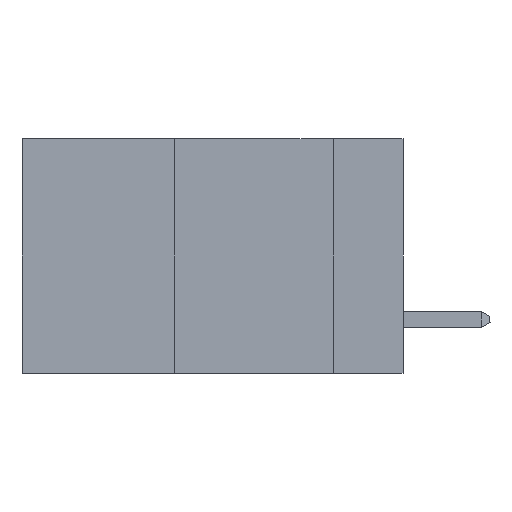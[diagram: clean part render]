
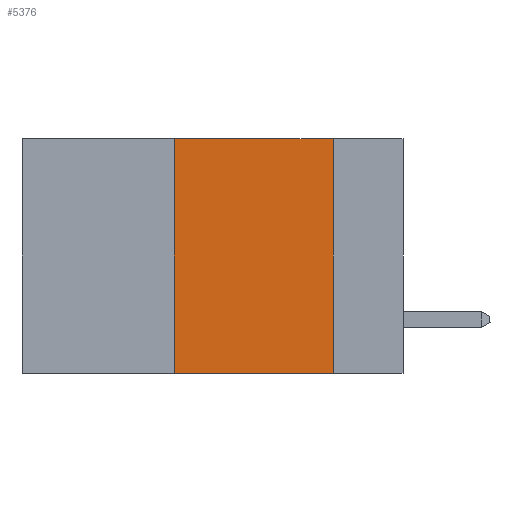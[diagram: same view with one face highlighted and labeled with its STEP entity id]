
A CAD part, left-side view. The second image highlights one B-rep face of the part: STEP entity #5376.
In plain terms, the highlighted planar face has unit normal (-1, 0, 0).
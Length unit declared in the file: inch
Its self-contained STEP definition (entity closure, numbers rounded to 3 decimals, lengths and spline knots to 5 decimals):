
#1169 = AXIS2_PLACEMENT_3D ( 'NONE', #4133, #14117, #9190 ) ;
#1533 = CARTESIAN_POINT ( 'NONE',  ( 0., 0.6, 0. ) ) ;
#1598 = VECTOR ( 'NONE', #25579, 39.37008 ) ;
#3193 = ORIENTED_EDGE ( 'NONE', *, *, #7996, .F. ) ;
#4133 = CARTESIAN_POINT ( 'NONE',  ( 0., 0.6, 0. ) ) ;
#5376 = ADVANCED_FACE ( 'NONE', ( #31578 ), #29357, .F. ) ;
#5491 = LINE ( 'NONE', #19817, #31745 ) ;
#7757 = CARTESIAN_POINT ( 'NONE',  ( 0., 0.36, 0. ) ) ;
#7996 = EDGE_CURVE ( 'NONE', #14707, #30590, #23059, .T. ) ;
#8188 = ORIENTED_EDGE ( 'NONE', *, *, #14630, .F. ) ;
#8896 = EDGE_CURVE ( 'NONE', #24119, #30255, #5491, .T. ) ;
#9190 = DIRECTION ( 'NONE',  ( 0., 0., -1. ) ) ;
#11296 = VECTOR ( 'NONE', #16432, 39.37008 ) ;
#12217 = ORIENTED_EDGE ( 'NONE', *, *, #16484, .T. ) ;
#12591 = DIRECTION ( 'NONE',  ( 0., -1., 0. ) ) ;
#13090 = CARTESIAN_POINT ( 'NONE',  ( 0., 0.36, 0. ) ) ;
#14106 = CARTESIAN_POINT ( 'NONE',  ( 0., 0.11, -0.37 ) ) ;
#14117 = DIRECTION ( 'NONE',  ( 1., 0., 0. ) ) ;
#14630 = EDGE_CURVE ( 'NONE', #30590, #24119, #18474, .T. ) ;
#14707 = VERTEX_POINT ( 'NONE', #19080 ) ;
#16432 = DIRECTION ( 'NONE',  ( 0., -1., 0. ) ) ;
#16484 = EDGE_CURVE ( 'NONE', #14707, #30255, #20738, .T. ) ;
#17288 = CARTESIAN_POINT ( 'NONE',  ( 0., 0.6, -0.37 ) ) ;
#18243 = ORIENTED_EDGE ( 'NONE', *, *, #8896, .F. ) ;
#18474 = LINE ( 'NONE', #1533, #11296 ) ;
#19080 = CARTESIAN_POINT ( 'NONE',  ( 0., 0.36, -0.37 ) ) ;
#19557 = EDGE_LOOP ( 'NONE', ( #18243, #8188, #3193, #12217 ) ) ;
#19817 = CARTESIAN_POINT ( 'NONE',  ( 0., 0.11, 0. ) ) ;
#20738 = LINE ( 'NONE', #17288, #24754 ) ;
#23059 = LINE ( 'NONE', #7757, #1598 ) ;
#23729 = CARTESIAN_POINT ( 'NONE',  ( 0., 0.11, 0. ) ) ;
#24119 = VERTEX_POINT ( 'NONE', #23729 ) ;
#24754 = VECTOR ( 'NONE', #12591, 39.37008 ) ;
#25579 = DIRECTION ( 'NONE',  ( 0., 0., 1. ) ) ;
#29191 = DIRECTION ( 'NONE',  ( 0., 0., -1. ) ) ;
#29357 = PLANE ( 'NONE',  #1169 ) ;
#30255 = VERTEX_POINT ( 'NONE', #14106 ) ;
#30590 = VERTEX_POINT ( 'NONE', #13090 ) ;
#31578 = FACE_OUTER_BOUND ( 'NONE', #19557, .T. ) ;
#31745 = VECTOR ( 'NONE', #29191, 39.37008 ) ;
